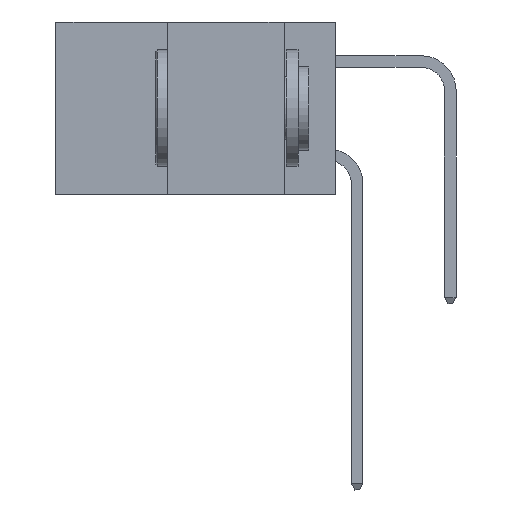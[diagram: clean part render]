
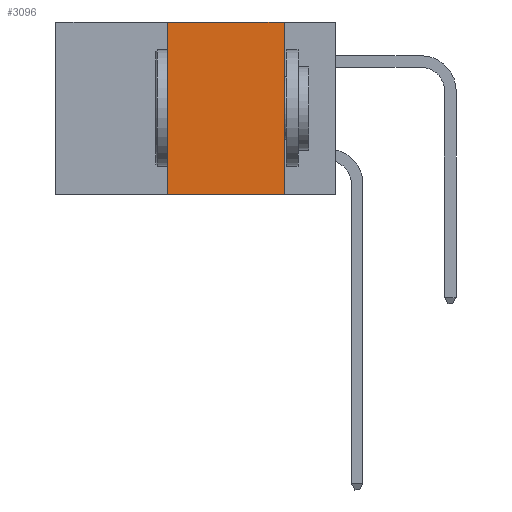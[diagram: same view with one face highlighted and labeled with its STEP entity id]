
A CAD part, left-side view. The second image highlights one B-rep face of the part: STEP entity #3096.
In plain terms, the highlighted planar face has unit normal (-1, 0, 0).
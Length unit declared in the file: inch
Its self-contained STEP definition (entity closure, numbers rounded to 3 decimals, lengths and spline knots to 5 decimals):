
#403 = CARTESIAN_POINT ( 'NONE',  ( 0., 0.6, -0.37 ) ) ;
#2269 = ORIENTED_EDGE ( 'NONE', *, *, #30430, .F. ) ;
#2491 = DIRECTION ( 'NONE',  ( 0., 0., 1. ) ) ;
#3096 = ADVANCED_FACE ( 'NONE', ( #21058 ), #5411, .F. ) ;
#3539 = EDGE_CURVE ( 'NONE', #11389, #6746, #40537, .T. ) ;
#3687 = LINE ( 'NONE', #31995, #12406 ) ;
#4223 = DIRECTION ( 'NONE',  ( 0., -1., 0. ) ) ;
#4986 = EDGE_LOOP ( 'NONE', ( #41964, #27656, #2269, #6980 ) ) ;
#5411 = PLANE ( 'NONE',  #33296 ) ;
#6526 = CARTESIAN_POINT ( 'NONE',  ( 0., 0.11, 0. ) ) ;
#6726 = VECTOR ( 'NONE', #19154, 39.37008 ) ;
#6746 = VERTEX_POINT ( 'NONE', #37402 ) ;
#6980 = ORIENTED_EDGE ( 'NONE', *, *, #3539, .T. ) ;
#7883 = LINE ( 'NONE', #8063, #6726 ) ;
#8063 = CARTESIAN_POINT ( 'NONE',  ( 0., 0.6, 0. ) ) ;
#8536 = EDGE_CURVE ( 'NONE', #16929, #29217, #7883, .T. ) ;
#8599 = CARTESIAN_POINT ( 'NONE',  ( 0., 0.36, 0. ) ) ;
#11250 = VECTOR ( 'NONE', #4223, 39.37008 ) ;
#11389 = VERTEX_POINT ( 'NONE', #34482 ) ;
#11503 = EDGE_CURVE ( 'NONE', #29217, #6746, #47382, .T. ) ;
#12406 = VECTOR ( 'NONE', #2491, 39.37008 ) ;
#12845 = DIRECTION ( 'NONE',  ( 0., 0., -1. ) ) ;
#16929 = VERTEX_POINT ( 'NONE', #8599 ) ;
#18085 = VECTOR ( 'NONE', #27764, 39.37008 ) ;
#19154 = DIRECTION ( 'NONE',  ( 0., -1., 0. ) ) ;
#21058 = FACE_OUTER_BOUND ( 'NONE', #4986, .T. ) ;
#27656 = ORIENTED_EDGE ( 'NONE', *, *, #8536, .F. ) ;
#27764 = DIRECTION ( 'NONE',  ( 0., 0., -1. ) ) ;
#29217 = VERTEX_POINT ( 'NONE', #6526 ) ;
#30430 = EDGE_CURVE ( 'NONE', #11389, #16929, #3687, .T. ) ;
#31995 = CARTESIAN_POINT ( 'NONE',  ( 0., 0.36, 0. ) ) ;
#33296 = AXIS2_PLACEMENT_3D ( 'NONE', #45768, #34822, #12845 ) ;
#34482 = CARTESIAN_POINT ( 'NONE',  ( 0., 0.36, -0.37 ) ) ;
#34822 = DIRECTION ( 'NONE',  ( 1., 0., 0. ) ) ;
#37402 = CARTESIAN_POINT ( 'NONE',  ( 0., 0.11, -0.37 ) ) ;
#40537 = LINE ( 'NONE', #403, #11250 ) ;
#41964 = ORIENTED_EDGE ( 'NONE', *, *, #11503, .F. ) ;
#42347 = CARTESIAN_POINT ( 'NONE',  ( 0., 0.11, 0. ) ) ;
#45768 = CARTESIAN_POINT ( 'NONE',  ( 0., 0.6, 0. ) ) ;
#47382 = LINE ( 'NONE', #42347, #18085 ) ;
